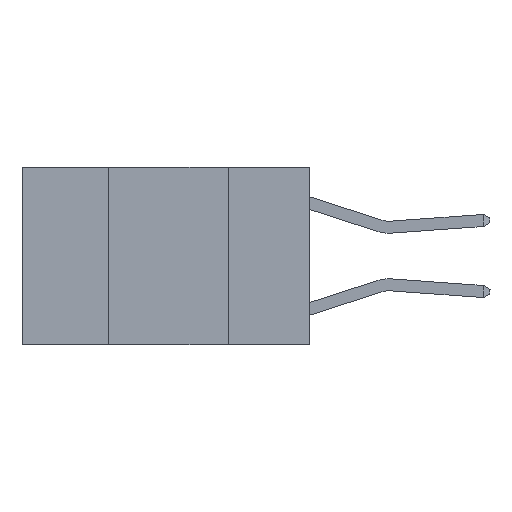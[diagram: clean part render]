
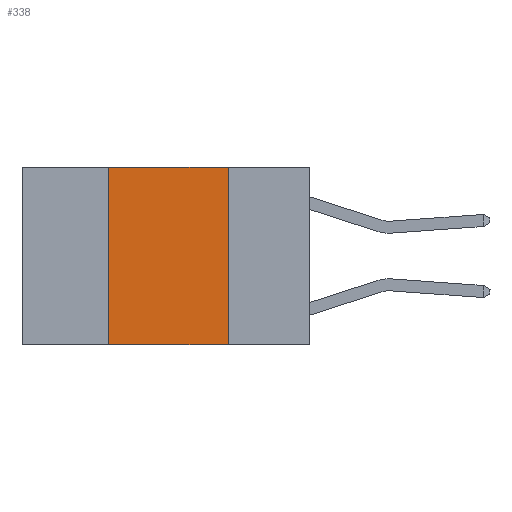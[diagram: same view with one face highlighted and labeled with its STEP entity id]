
A CAD part, left-side view. The second image highlights one B-rep face of the part: STEP entity #338.
In plain terms, the highlighted planar face has unit normal (-1, 0, 0).
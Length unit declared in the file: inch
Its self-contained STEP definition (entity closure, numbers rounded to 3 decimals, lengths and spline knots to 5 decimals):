
#338 = ADVANCED_FACE ( 'NONE', ( #4035 ), #4016, .F. ) ;
#653 = CARTESIAN_POINT ( 'NONE',  ( 0., 0.42, 0. ) ) ;
#2292 = VECTOR ( 'NONE', #15594, 39.37008 ) ;
#2576 = CARTESIAN_POINT ( 'NONE',  ( 0., 0.17, 0. ) ) ;
#2816 = LINE ( 'NONE', #2576, #13257 ) ;
#2823 = DIRECTION ( 'NONE',  ( 1., 0., 0. ) ) ;
#3713 = LINE ( 'NONE', #9898, #9493 ) ;
#3775 = DIRECTION ( 'NONE',  ( 0., -1., 0. ) ) ;
#4016 = PLANE ( 'NONE',  #13557 ) ;
#4035 = FACE_OUTER_BOUND ( 'NONE', #8794, .T. ) ;
#4474 = CARTESIAN_POINT ( 'NONE',  ( 0., 0.6, 0. ) ) ;
#5209 = ORIENTED_EDGE ( 'NONE', *, *, #8863, .F. ) ;
#5628 = EDGE_CURVE ( 'NONE', #10960, #12057, #5648, .T. ) ;
#5648 = LINE ( 'NONE', #7284, #2292 ) ;
#5972 = CARTESIAN_POINT ( 'NONE',  ( 0., 0.42, 0. ) ) ;
#6414 = CARTESIAN_POINT ( 'NONE',  ( 0., 0.17, 0. ) ) ;
#6717 = LINE ( 'NONE', #653, #12697 ) ;
#7006 = DIRECTION ( 'NONE',  ( 0., 0., 1. ) ) ;
#7284 = CARTESIAN_POINT ( 'NONE',  ( 0., 0.6, -0.37 ) ) ;
#8080 = EDGE_CURVE ( 'NONE', #8464, #12057, #2816, .T. ) ;
#8464 = VERTEX_POINT ( 'NONE', #6414 ) ;
#8794 = EDGE_LOOP ( 'NONE', ( #10844, #11242, #5209, #11975 ) ) ;
#8863 = EDGE_CURVE ( 'NONE', #10960, #9004, #6717, .T. ) ;
#9004 = VERTEX_POINT ( 'NONE', #5972 ) ;
#9493 = VECTOR ( 'NONE', #3775, 39.37008 ) ;
#9898 = CARTESIAN_POINT ( 'NONE',  ( 0., 0.6, 0. ) ) ;
#10030 = DIRECTION ( 'NONE',  ( 0., 0., -1. ) ) ;
#10031 = EDGE_CURVE ( 'NONE', #9004, #8464, #3713, .T. ) ;
#10844 = ORIENTED_EDGE ( 'NONE', *, *, #8080, .F. ) ;
#10951 = CARTESIAN_POINT ( 'NONE',  ( 0., 0.17, -0.37 ) ) ;
#10960 = VERTEX_POINT ( 'NONE', #13616 ) ;
#11152 = DIRECTION ( 'NONE',  ( 0., 0., -1. ) ) ;
#11242 = ORIENTED_EDGE ( 'NONE', *, *, #10031, .F. ) ;
#11975 = ORIENTED_EDGE ( 'NONE', *, *, #5628, .T. ) ;
#12057 = VERTEX_POINT ( 'NONE', #10951 ) ;
#12697 = VECTOR ( 'NONE', #7006, 39.37008 ) ;
#13257 = VECTOR ( 'NONE', #11152, 39.37008 ) ;
#13557 = AXIS2_PLACEMENT_3D ( 'NONE', #4474, #2823, #10030 ) ;
#13616 = CARTESIAN_POINT ( 'NONE',  ( 0., 0.42, -0.37 ) ) ;
#15594 = DIRECTION ( 'NONE',  ( 0., -1., 0. ) ) ;
